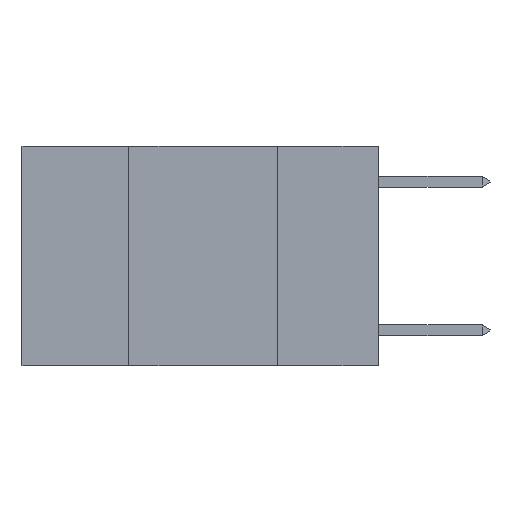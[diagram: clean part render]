
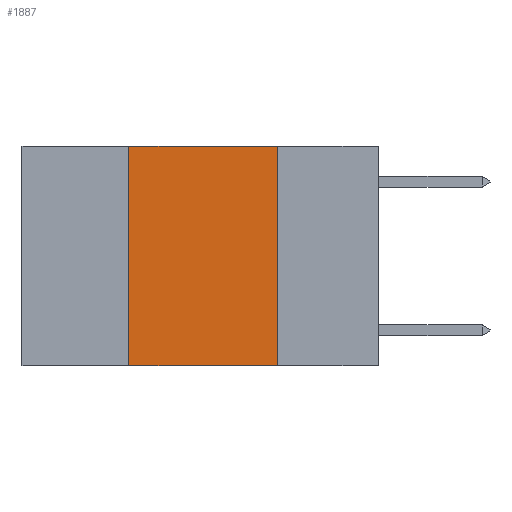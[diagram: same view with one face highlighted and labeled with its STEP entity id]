
A CAD part, left-side view. The second image highlights one B-rep face of the part: STEP entity #1887.
In plain terms, the highlighted planar face has unit normal (-1, 0, 0).
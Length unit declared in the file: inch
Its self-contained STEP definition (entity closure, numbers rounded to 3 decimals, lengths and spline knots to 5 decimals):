
#315 = VERTEX_POINT ( 'NONE', #8411 ) ;
#449 = AXIS2_PLACEMENT_3D ( 'NONE', #8008, #3301, #10066 ) ;
#1162 = VERTEX_POINT ( 'NONE', #10283 ) ;
#1250 = CARTESIAN_POINT ( 'NONE',  ( 0., 0.42, -0.37 ) ) ;
#1887 = ADVANCED_FACE ( 'NONE', ( #3364 ), #10941, .F. ) ;
#2061 = VECTOR ( 'NONE', #2358, 39.37008 ) ;
#2302 = CARTESIAN_POINT ( 'NONE',  ( 0., 0.6, -0.37 ) ) ;
#2358 = DIRECTION ( 'NONE',  ( 0., -1., 0. ) ) ;
#2425 = LINE ( 'NONE', #2302, #2061 ) ;
#2821 = EDGE_LOOP ( 'NONE', ( #3840, #10793, #3764, #8635 ) ) ;
#3294 = DIRECTION ( 'NONE',  ( 0., -1., 0. ) ) ;
#3301 = DIRECTION ( 'NONE',  ( 1., 0., 0. ) ) ;
#3364 = FACE_OUTER_BOUND ( 'NONE', #2821, .T. ) ;
#3764 = ORIENTED_EDGE ( 'NONE', *, *, #5489, .F. ) ;
#3798 = EDGE_CURVE ( 'NONE', #11568, #9724, #2425, .T. ) ;
#3840 = ORIENTED_EDGE ( 'NONE', *, *, #7021, .F. ) ;
#5460 = EDGE_CURVE ( 'NONE', #315, #1162, #12053, .T. ) ;
#5489 = EDGE_CURVE ( 'NONE', #11568, #315, #11309, .T. ) ;
#5787 = VECTOR ( 'NONE', #11248, 39.37008 ) ;
#5976 = VECTOR ( 'NONE', #3294, 39.37008 ) ;
#6373 = VECTOR ( 'NONE', #10390, 39.37008 ) ;
#7021 = EDGE_CURVE ( 'NONE', #1162, #9724, #10502, .T. ) ;
#8008 = CARTESIAN_POINT ( 'NONE',  ( 0., 0.6, 0. ) ) ;
#8411 = CARTESIAN_POINT ( 'NONE',  ( 0., 0.42, 0. ) ) ;
#8635 = ORIENTED_EDGE ( 'NONE', *, *, #3798, .T. ) ;
#9724 = VERTEX_POINT ( 'NONE', #11472 ) ;
#10066 = DIRECTION ( 'NONE',  ( 0., 0., -1. ) ) ;
#10283 = CARTESIAN_POINT ( 'NONE',  ( 0., 0.17, 0. ) ) ;
#10390 = DIRECTION ( 'NONE',  ( 0., 0., -1. ) ) ;
#10502 = LINE ( 'NONE', #11503, #6373 ) ;
#10793 = ORIENTED_EDGE ( 'NONE', *, *, #5460, .F. ) ;
#10941 = PLANE ( 'NONE',  #449 ) ;
#11052 = CARTESIAN_POINT ( 'NONE',  ( 0., 0.6, 0. ) ) ;
#11248 = DIRECTION ( 'NONE',  ( 0., 0., 1. ) ) ;
#11309 = LINE ( 'NONE', #11441, #5787 ) ;
#11441 = CARTESIAN_POINT ( 'NONE',  ( 0., 0.42, 0. ) ) ;
#11472 = CARTESIAN_POINT ( 'NONE',  ( 0., 0.17, -0.37 ) ) ;
#11503 = CARTESIAN_POINT ( 'NONE',  ( 0., 0.17, 0. ) ) ;
#11568 = VERTEX_POINT ( 'NONE', #1250 ) ;
#12053 = LINE ( 'NONE', #11052, #5976 ) ;
